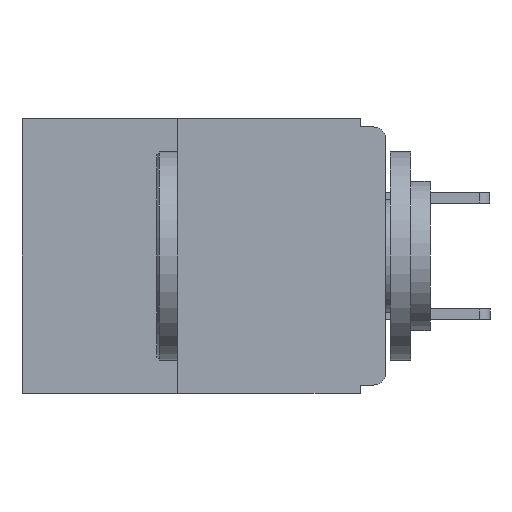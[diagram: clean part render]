
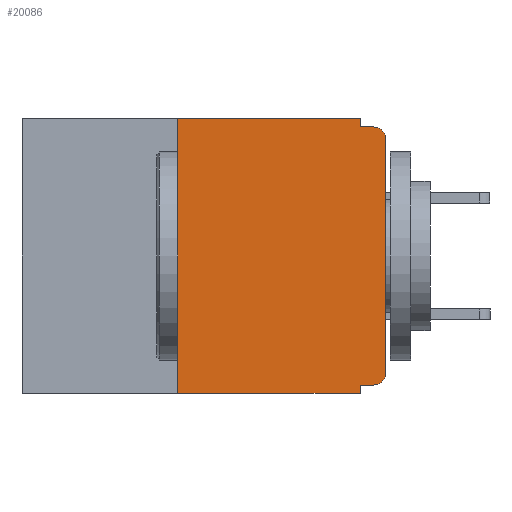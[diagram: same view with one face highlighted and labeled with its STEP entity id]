
A CAD part, left-side view. The second image highlights one B-rep face of the part: STEP entity #20086.
In plain terms, the highlighted planar face has unit normal (-1, 0, 0).
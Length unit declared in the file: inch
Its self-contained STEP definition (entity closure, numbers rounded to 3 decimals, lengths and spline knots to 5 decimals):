
#165 = AXIS2_PLACEMENT_3D ( 'NONE', #18605, #6456, #20599 ) ;
#196 = CARTESIAN_POINT ( 'NONE',  ( 0., 0., -0.305 ) ) ;
#631 = EDGE_CURVE ( 'NONE', #19075, #5483, #10176, .T. ) ;
#647 = CARTESIAN_POINT ( 'NONE',  ( 0., 0.437, 0. ) ) ;
#1770 = VERTEX_POINT ( 'NONE', #196 ) ;
#2715 = DIRECTION ( 'NONE',  ( 0., 0., -1. ) ) ;
#3129 = EDGE_CURVE ( 'NONE', #6117, #6000, #12622, .T. ) ;
#3790 = CARTESIAN_POINT ( 'NONE',  ( 0., 0., -0.025 ) ) ;
#4152 = VECTOR ( 'NONE', #15630, 39.37008 ) ;
#4384 = LINE ( 'NONE', #13564, #20533 ) ;
#4477 = EDGE_CURVE ( 'NONE', #16660, #6000, #7130, .T. ) ;
#5075 = VECTOR ( 'NONE', #10808, 39.37008 ) ;
#5366 = CARTESIAN_POINT ( 'NONE',  ( 0., 0.437, 0. ) ) ;
#5483 = VERTEX_POINT ( 'NONE', #16254 ) ;
#5695 = EDGE_CURVE ( 'NONE', #13352, #11072, #24317, .T. ) ;
#5737 = LINE ( 'NONE', #10837, #5075 ) ;
#5851 = EDGE_CURVE ( 'NONE', #16660, #19075, #5737, .T. ) ;
#5948 = CARTESIAN_POINT ( 'NONE',  ( 0., 0.015, -0.305 ) ) ;
#6000 = VERTEX_POINT ( 'NONE', #8979 ) ;
#6117 = VERTEX_POINT ( 'NONE', #7046 ) ;
#6145 = AXIS2_PLACEMENT_3D ( 'NONE', #5948, #20111, #7988 ) ;
#6456 = DIRECTION ( 'NONE',  ( -1., 0., 0. ) ) ;
#6843 = VERTEX_POINT ( 'NONE', #3790 ) ;
#6853 = LINE ( 'NONE', #23214, #7497 ) ;
#6998 = AXIS2_PLACEMENT_3D ( 'NONE', #647, #14925, #2715 ) ;
#7046 = CARTESIAN_POINT ( 'NONE',  ( 0., 0.031, -0.32 ) ) ;
#7130 = LINE ( 'NONE', #19512, #7759 ) ;
#7224 = EDGE_CURVE ( 'NONE', #5483, #13352, #4384, .T. ) ;
#7497 = VECTOR ( 'NONE', #25128, 39.37008 ) ;
#7759 = VECTOR ( 'NONE', #18696, 39.37008 ) ;
#7988 = DIRECTION ( 'NONE',  ( 0., 0., -1. ) ) ;
#8979 = CARTESIAN_POINT ( 'NONE',  ( 0., 0.031, -0.33 ) ) ;
#9628 = VERTEX_POINT ( 'NONE', #17308 ) ;
#10033 = VECTOR ( 'NONE', #23247, 39.37008 ) ;
#10176 = LINE ( 'NONE', #5366, #4152 ) ;
#10428 = CARTESIAN_POINT ( 'NONE',  ( 0., 0.25, 0. ) ) ;
#10665 = LINE ( 'NONE', #15227, #10033 ) ;
#10808 = DIRECTION ( 'NONE',  ( 0., 0., 1. ) ) ;
#10837 = CARTESIAN_POINT ( 'NONE',  ( 0., 0.25, -0.33 ) ) ;
#11072 = VERTEX_POINT ( 'NONE', #12428 ) ;
#12428 = CARTESIAN_POINT ( 'NONE',  ( 0., 0.015, -0.01 ) ) ;
#12526 = EDGE_CURVE ( 'NONE', #1770, #6843, #6853, .T. ) ;
#12622 = LINE ( 'NONE', #22872, #22649 ) ;
#12980 = DIRECTION ( 'NONE',  ( 0., -1., 0. ) ) ;
#13075 = CARTESIAN_POINT ( 'NONE',  ( 0., 0., -0.01 ) ) ;
#13157 = ORIENTED_EDGE ( 'NONE', *, *, #12526, .T. ) ;
#13182 = ORIENTED_EDGE ( 'NONE', *, *, #22427, .T. ) ;
#13352 = VERTEX_POINT ( 'NONE', #17972 ) ;
#13462 = ORIENTED_EDGE ( 'NONE', *, *, #5695, .F. ) ;
#13469 = DIRECTION ( 'NONE',  ( 0., 0., -1. ) ) ;
#13564 = CARTESIAN_POINT ( 'NONE',  ( 0., 0.031, 0. ) ) ;
#13646 = ORIENTED_EDGE ( 'NONE', *, *, #7224, .F. ) ;
#13742 = VECTOR ( 'NONE', #12980, 39.37008 ) ;
#13770 = ORIENTED_EDGE ( 'NONE', *, *, #631, .F. ) ;
#14498 = ORIENTED_EDGE ( 'NONE', *, *, #5851, .F. ) ;
#14925 = DIRECTION ( 'NONE',  ( 1., 0., 0. ) ) ;
#15227 = CARTESIAN_POINT ( 'NONE',  ( 0., 0., -0.32 ) ) ;
#15494 = ORIENTED_EDGE ( 'NONE', *, *, #4477, .T. ) ;
#15599 = ORIENTED_EDGE ( 'NONE', *, *, #3129, .F. ) ;
#15630 = DIRECTION ( 'NONE',  ( 0., -1., 0. ) ) ;
#16047 = ORIENTED_EDGE ( 'NONE', *, *, #25011, .F. ) ;
#16101 = ORIENTED_EDGE ( 'NONE', *, *, #19788, .T. ) ;
#16254 = CARTESIAN_POINT ( 'NONE',  ( 0., 0.031, 0. ) ) ;
#16660 = VERTEX_POINT ( 'NONE', #18534 ) ;
#16945 = DIRECTION ( 'NONE',  ( 0., 0., -1. ) ) ;
#17308 = CARTESIAN_POINT ( 'NONE',  ( 0., 0.015, -0.32 ) ) ;
#17792 = CIRCLE ( 'NONE', #165, 0.015 ) ;
#17972 = CARTESIAN_POINT ( 'NONE',  ( 0., 0.031, -0.01 ) ) ;
#18534 = CARTESIAN_POINT ( 'NONE',  ( 0., 0.25, -0.33 ) ) ;
#18605 = CARTESIAN_POINT ( 'NONE',  ( 0., 0.015, -0.025 ) ) ;
#18696 = DIRECTION ( 'NONE',  ( 0., -1., 0. ) ) ;
#19075 = VERTEX_POINT ( 'NONE', #10428 ) ;
#19512 = CARTESIAN_POINT ( 'NONE',  ( 0., 0.437, -0.33 ) ) ;
#19724 = EDGE_LOOP ( 'NONE', ( #13157, #13182, #13462, #13646, #13770, #14498, #15494, #15599, #16047, #16101 ) ) ;
#19788 = EDGE_CURVE ( 'NONE', #9628, #1770, #20720, .T. ) ;
#20086 = ADVANCED_FACE ( 'NONE', ( #24978 ), #24801, .F. ) ;
#20111 = DIRECTION ( 'NONE',  ( -1., 0., 0. ) ) ;
#20533 = VECTOR ( 'NONE', #13469, 39.37008 ) ;
#20599 = DIRECTION ( 'NONE',  ( 0., 0., -1. ) ) ;
#20720 = CIRCLE ( 'NONE', #6145, 0.015 ) ;
#22427 = EDGE_CURVE ( 'NONE', #6843, #11072, #17792, .T. ) ;
#22649 = VECTOR ( 'NONE', #16945, 39.37008 ) ;
#22872 = CARTESIAN_POINT ( 'NONE',  ( 0., 0.031, -0.33 ) ) ;
#23214 = CARTESIAN_POINT ( 'NONE',  ( 0., 0., 0. ) ) ;
#23247 = DIRECTION ( 'NONE',  ( 0., 1., 0. ) ) ;
#24317 = LINE ( 'NONE', #13075, #13742 ) ;
#24801 = PLANE ( 'NONE',  #6998 ) ;
#24978 = FACE_OUTER_BOUND ( 'NONE', #19724, .T. ) ;
#25011 = EDGE_CURVE ( 'NONE', #9628, #6117, #10665, .T. ) ;
#25128 = DIRECTION ( 'NONE',  ( 0., 0., 1. ) ) ;
